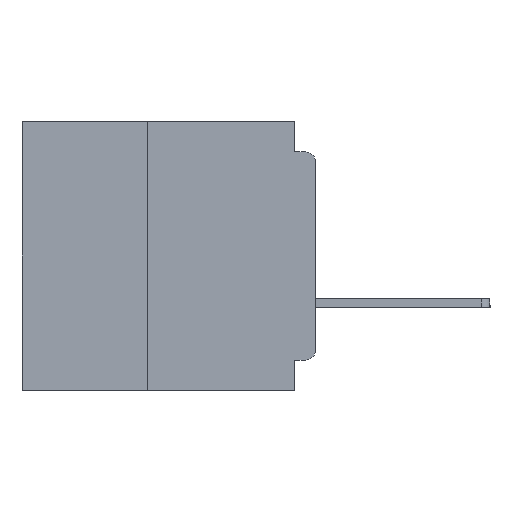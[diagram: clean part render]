
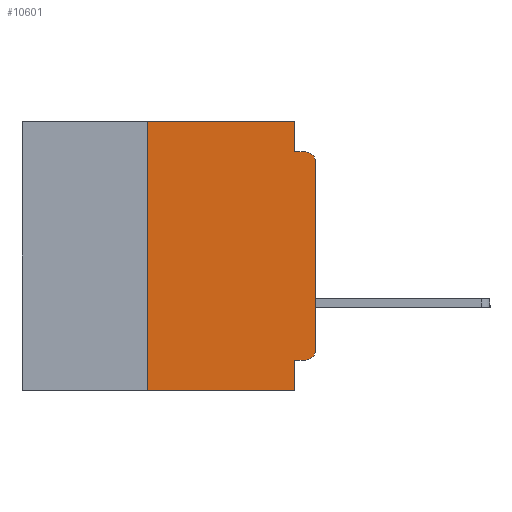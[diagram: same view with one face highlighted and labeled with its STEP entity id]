
A CAD part, left-side view. The second image highlights one B-rep face of the part: STEP entity #10601.
In plain terms, the highlighted planar face has unit normal (-1, 0, 0).
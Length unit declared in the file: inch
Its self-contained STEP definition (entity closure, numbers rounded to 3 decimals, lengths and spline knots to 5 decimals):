
#1335 = VERTEX_POINT ( 'NONE', #52874 ) ;
#1362 = ORIENTED_EDGE ( 'NONE', *, *, #4042, .T. ) ;
#1641 = CIRCLE ( 'NONE', #16088, 0.015 ) ;
#1704 = ORIENTED_EDGE ( 'NONE', *, *, #47754, .F. ) ;
#2735 = CARTESIAN_POINT ( 'NONE',  ( 0., 0.437, 0. ) ) ;
#4042 = EDGE_CURVE ( 'NONE', #1335, #14188, #18004, .T. ) ;
#4531 = EDGE_CURVE ( 'NONE', #38080, #14188, #48484, .T. ) ;
#5454 = VECTOR ( 'NONE', #9921, 39.37008 ) ;
#6148 = DIRECTION ( 'NONE',  ( -1., 0., 0. ) ) ;
#6457 = VERTEX_POINT ( 'NONE', #10831 ) ;
#7768 = AXIS2_PLACEMENT_3D ( 'NONE', #2735, #36228, #11339 ) ;
#7855 = ORIENTED_EDGE ( 'NONE', *, *, #45208, .F. ) ;
#8173 = CARTESIAN_POINT ( 'NONE',  ( 0., 0.015, -0.045 ) ) ;
#8195 = CARTESIAN_POINT ( 'NONE',  ( 0., 0., -0.34 ) ) ;
#8326 = EDGE_CURVE ( 'NONE', #34167, #39003, #1641, .T. ) ;
#8582 = DIRECTION ( 'NONE',  ( 0., 0., -1. ) ) ;
#8826 = VERTEX_POINT ( 'NONE', #40784 ) ;
#9040 = VECTOR ( 'NONE', #51797, 39.37008 ) ;
#9921 = DIRECTION ( 'NONE',  ( 0., 0., -1. ) ) ;
#10244 = VERTEX_POINT ( 'NONE', #8195 ) ;
#10601 = ADVANCED_FACE ( 'NONE', ( #30353 ), #52645, .F. ) ;
#10831 = CARTESIAN_POINT ( 'NONE',  ( 0., 0.015, -0.355 ) ) ;
#10995 = DIRECTION ( 'NONE',  ( 0., -1., 0. ) ) ;
#11339 = DIRECTION ( 'NONE',  ( 0., 0., -1. ) ) ;
#11637 = CARTESIAN_POINT ( 'NONE',  ( 0., 0., -0.06 ) ) ;
#13068 = EDGE_CURVE ( 'NONE', #37872, #39003, #46540, .T. ) ;
#13469 = EDGE_CURVE ( 'NONE', #6457, #10244, #36784, .T. ) ;
#14188 = VERTEX_POINT ( 'NONE', #22808 ) ;
#15195 = ORIENTED_EDGE ( 'NONE', *, *, #51267, .T. ) ;
#16088 = AXIS2_PLACEMENT_3D ( 'NONE', #31151, #6148, #35330 ) ;
#16410 = LINE ( 'NONE', #49002, #24831 ) ;
#16513 = CARTESIAN_POINT ( 'NONE',  ( 0., 0.031, -0.045 ) ) ;
#17773 = CARTESIAN_POINT ( 'NONE',  ( 0., 0.031, -0.355 ) ) ;
#17852 = CARTESIAN_POINT ( 'NONE',  ( 0., 0.015, -0.34 ) ) ;
#18004 = LINE ( 'NONE', #52205, #51088 ) ;
#19123 = VECTOR ( 'NONE', #19349, 39.37008 ) ;
#19222 = AXIS2_PLACEMENT_3D ( 'NONE', #17852, #46906, #21986 ) ;
#19349 = DIRECTION ( 'NONE',  ( 0., 0., 1. ) ) ;
#20751 = CARTESIAN_POINT ( 'NONE',  ( 0., 0.031, 0. ) ) ;
#20961 = DIRECTION ( 'NONE',  ( 0., 1., 0. ) ) ;
#21986 = DIRECTION ( 'NONE',  ( 0., 0., -1. ) ) ;
#22808 = CARTESIAN_POINT ( 'NONE',  ( 0., 0.031, -0.4 ) ) ;
#23361 = ORIENTED_EDGE ( 'NONE', *, *, #50258, .F. ) ;
#24831 = VECTOR ( 'NONE', #53093, 39.37008 ) ;
#24984 = LINE ( 'NONE', #29009, #45793 ) ;
#27933 = ORIENTED_EDGE ( 'NONE', *, *, #4531, .F. ) ;
#29009 = CARTESIAN_POINT ( 'NONE',  ( 0., 0., -0.355 ) ) ;
#30353 = FACE_OUTER_BOUND ( 'NONE', #32972, .T. ) ;
#30663 = LINE ( 'NONE', #20751, #39161 ) ;
#31151 = CARTESIAN_POINT ( 'NONE',  ( 0., 0.015, -0.06 ) ) ;
#32972 = EDGE_LOOP ( 'NONE', ( #15195, #35730, #50591, #23361, #7855, #53448, #1362, #27933, #1704, #48924 ) ) ;
#34167 = VERTEX_POINT ( 'NONE', #11637 ) ;
#34229 = CARTESIAN_POINT ( 'NONE',  ( 0., 0.25, 0. ) ) ;
#35103 = VERTEX_POINT ( 'NONE', #34229 ) ;
#35330 = DIRECTION ( 'NONE',  ( 0., 0., -1. ) ) ;
#35506 = VECTOR ( 'NONE', #10995, 39.37008 ) ;
#35730 = ORIENTED_EDGE ( 'NONE', *, *, #8326, .T. ) ;
#36228 = DIRECTION ( 'NONE',  ( 1., 0., 0. ) ) ;
#36784 = CIRCLE ( 'NONE', #19222, 0.015 ) ;
#37872 = VERTEX_POINT ( 'NONE', #16513 ) ;
#38080 = VERTEX_POINT ( 'NONE', #17773 ) ;
#39003 = VERTEX_POINT ( 'NONE', #8173 ) ;
#39033 = CARTESIAN_POINT ( 'NONE',  ( 0., 0.031, -0.4 ) ) ;
#39161 = VECTOR ( 'NONE', #8582, 39.37008 ) ;
#39814 = DIRECTION ( 'NONE',  ( 0., -1., 0. ) ) ;
#40104 = CARTESIAN_POINT ( 'NONE',  ( 0., 0., -0.045 ) ) ;
#40784 = CARTESIAN_POINT ( 'NONE',  ( 0., 0.031, 0. ) ) ;
#41051 = EDGE_CURVE ( 'NONE', #1335, #35103, #50933, .T. ) ;
#42260 = LINE ( 'NONE', #47683, #9040 ) ;
#44256 = CARTESIAN_POINT ( 'NONE',  ( 0., 0.25, -0.4 ) ) ;
#45208 = EDGE_CURVE ( 'NONE', #35103, #8826, #16410, .T. ) ;
#45793 = VECTOR ( 'NONE', #20961, 39.37008 ) ;
#46540 = LINE ( 'NONE', #40104, #35506 ) ;
#46906 = DIRECTION ( 'NONE',  ( -1., 0., 0. ) ) ;
#47683 = CARTESIAN_POINT ( 'NONE',  ( 0., 0., 0. ) ) ;
#47754 = EDGE_CURVE ( 'NONE', #6457, #38080, #24984, .T. ) ;
#48484 = LINE ( 'NONE', #39033, #5454 ) ;
#48924 = ORIENTED_EDGE ( 'NONE', *, *, #13469, .T. ) ;
#49002 = CARTESIAN_POINT ( 'NONE',  ( 0., 0.437, 0. ) ) ;
#50258 = EDGE_CURVE ( 'NONE', #8826, #37872, #30663, .T. ) ;
#50591 = ORIENTED_EDGE ( 'NONE', *, *, #13068, .F. ) ;
#50933 = LINE ( 'NONE', #44256, #19123 ) ;
#51088 = VECTOR ( 'NONE', #39814, 39.37008 ) ;
#51267 = EDGE_CURVE ( 'NONE', #10244, #34167, #42260, .T. ) ;
#51797 = DIRECTION ( 'NONE',  ( 0., 0., 1. ) ) ;
#52205 = CARTESIAN_POINT ( 'NONE',  ( 0., 0.437, -0.4 ) ) ;
#52645 = PLANE ( 'NONE',  #7768 ) ;
#52874 = CARTESIAN_POINT ( 'NONE',  ( 0., 0.25, -0.4 ) ) ;
#53093 = DIRECTION ( 'NONE',  ( 0., -1., 0. ) ) ;
#53448 = ORIENTED_EDGE ( 'NONE', *, *, #41051, .F. ) ;
